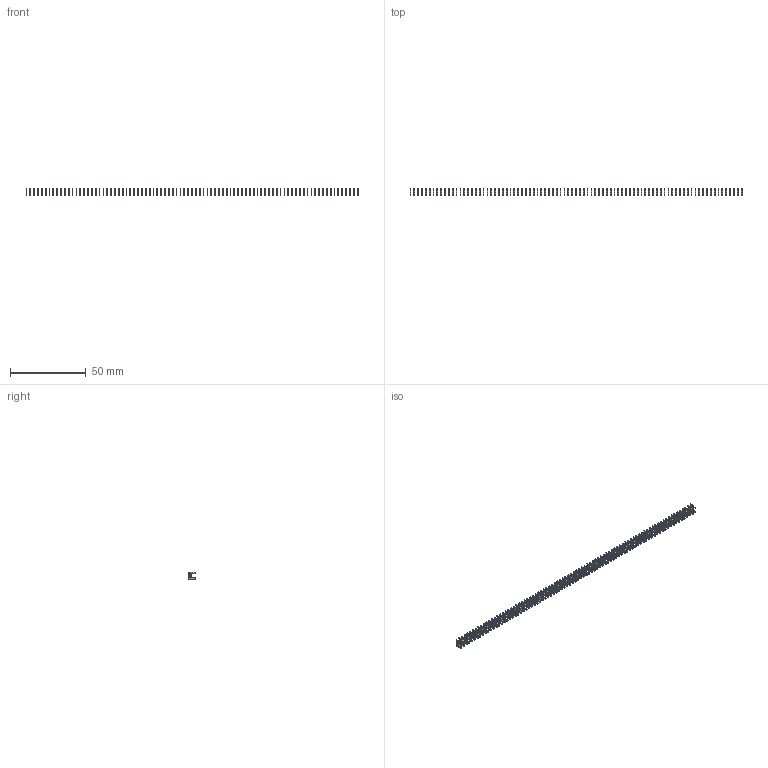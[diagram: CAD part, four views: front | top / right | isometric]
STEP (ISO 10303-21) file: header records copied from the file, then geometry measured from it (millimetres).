
FILE_DESCRIPTION (( 'STEP AP203' ), '1' );
FILE_NAME ('105-087-208-100.STEP', '2020-04-08T01:11:09', ( '' ), ( '' ), 'SwSTEP 2.0', 'SolidWorks 2016', '' );
FILE_SCHEMA (( 'CONFIG_CONTROL_DESIGN' ));
Length unit declared in the file: inch
Products named in the file (2): 105-087-208-100; 100-290-001_100-290-208
Assembly tree (87 placements, depth 2):
  105-087-208-100
    100-290-001_100-290-208  x87
Bounding box: 218.95 x 4.83 x 5.17 mm (x, y, z)
Volume: 598.6 mm3; surface area: 3697.2 mm2
Topology: 87 solids, 87 shells, 2175 faces, 6003 edges, 4002 vertices
Faces by surface type: plane 1914, cylinder 261
Entity records: 3741 total; most frequent: DIRECTION 305, CARTESIAN_POINT 230, CALENDAR_DATE 184, LOCAL_TIME 184, DATE_AND_TIME 184, COORDINATED_UNIVERSAL_TIME_OFFSET 184, ORIENTED_EDGE 138, AXIS2_PLACEMENT_3D 121
